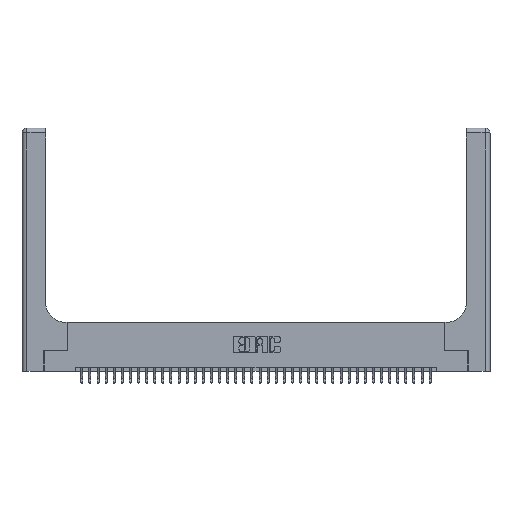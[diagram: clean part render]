
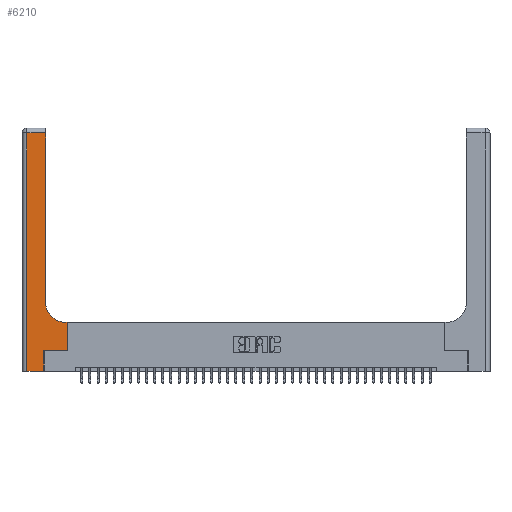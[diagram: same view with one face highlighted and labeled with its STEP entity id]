
A CAD part, top view. The second image highlights one B-rep face of the part: STEP entity #6210.
In plain terms, the highlighted planar face has unit normal (0, 0, 1).
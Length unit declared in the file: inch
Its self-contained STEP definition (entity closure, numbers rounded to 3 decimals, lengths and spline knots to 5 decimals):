
#316 = VERTEX_POINT ( 'NONE', #25435 ) ;
#557 = LINE ( 'NONE', #10463, #8726 ) ;
#2106 = CARTESIAN_POINT ( 'NONE',  ( 0.06, 3., 0.37 ) ) ;
#2370 = VECTOR ( 'NONE', #38681, 39.37008 ) ;
#2561 = VECTOR ( 'NONE', #31526, 39.37008 ) ;
#3027 = LINE ( 'NONE', #12879, #2561 ) ;
#3917 = ORIENTED_EDGE ( 'NONE', *, *, #30613, .T. ) ;
#4060 = LINE ( 'NONE', #8779, #21271 ) ;
#4466 = LINE ( 'NONE', #23834, #31785 ) ;
#4567 = DIRECTION ( 'NONE',  ( 0., 0., -1. ) ) ;
#6210 = ADVANCED_FACE ( 'NONE', ( #14023 ), #31458, .F. ) ;
#7527 = AXIS2_PLACEMENT_3D ( 'NONE', #19779, #16743, #13619 ) ;
#8027 = ORIENTED_EDGE ( 'NONE', *, *, #34618, .T. ) ;
#8530 = LINE ( 'NONE', #2106, #27703 ) ;
#8726 = VECTOR ( 'NONE', #35200, 39.37008 ) ;
#8779 = CARTESIAN_POINT ( 'NONE',  ( 0.5585, 0.25, 0.37 ) ) ;
#10171 = ORIENTED_EDGE ( 'NONE', *, *, #37333, .T. ) ;
#10463 = CARTESIAN_POINT ( 'NONE',  ( 0., 0., 0.37 ) ) ;
#10995 = DIRECTION ( 'NONE',  ( -1., 0., 0. ) ) ;
#11911 = ORIENTED_EDGE ( 'NONE', *, *, #30349, .T. ) ;
#12368 = VERTEX_POINT ( 'NONE', #21146 ) ;
#12558 = ORIENTED_EDGE ( 'NONE', *, *, #20154, .T. ) ;
#12695 = CARTESIAN_POINT ( 'NONE',  ( 0.5415, 0.6, 0.37 ) ) ;
#12879 = CARTESIAN_POINT ( 'NONE',  ( 0.269, 0., 0.37 ) ) ;
#13619 = DIRECTION ( 'NONE',  ( -1., 0., 0. ) ) ;
#14023 = FACE_OUTER_BOUND ( 'NONE', #19546, .T. ) ;
#14408 = CIRCLE ( 'NONE', #24457, 0.25 ) ;
#14654 = EDGE_CURVE ( 'NONE', #17067, #18882, #30308, .T. ) ;
#14672 = DIRECTION ( 'NONE',  ( 1., 0., 0. ) ) ;
#14797 = EDGE_CURVE ( 'NONE', #36912, #17067, #4466, .T. ) ;
#15057 = DIRECTION ( 'NONE',  ( 0., 1., 0. ) ) ;
#16743 = DIRECTION ( 'NONE',  ( 0., 0., -1. ) ) ;
#17067 = VERTEX_POINT ( 'NONE', #37466 ) ;
#17368 = VECTOR ( 'NONE', #14672, 39.37008 ) ;
#18251 = LINE ( 'NONE', #20681, #17368 ) ;
#18882 = VERTEX_POINT ( 'NONE', #34755 ) ;
#19546 = EDGE_LOOP ( 'NONE', ( #25445, #22291, #8027, #10171, #3917, #23276, #11911, #38232, #12558 ) ) ;
#19779 = CARTESIAN_POINT ( 'NONE',  ( 0., 3., 0.37 ) ) ;
#20090 = CARTESIAN_POINT ( 'NONE',  ( 0., 2.94, 0.37 ) ) ;
#20154 = EDGE_CURVE ( 'NONE', #34260, #36912, #14408, .T. ) ;
#20339 = CARTESIAN_POINT ( 'NONE',  ( 0.2915, 0.6, 0.37 ) ) ;
#20644 = EDGE_CURVE ( 'NONE', #29017, #34260, #29712, .T. ) ;
#20681 = CARTESIAN_POINT ( 'NONE',  ( 0.269, 0.25, 0.37 ) ) ;
#21146 = CARTESIAN_POINT ( 'NONE',  ( 0.06, 0., 0.37 ) ) ;
#21271 = VECTOR ( 'NONE', #15057, 39.37008 ) ;
#22291 = ORIENTED_EDGE ( 'NONE', *, *, #14654, .T. ) ;
#23117 = VECTOR ( 'NONE', #10995, 39.37008 ) ;
#23276 = ORIENTED_EDGE ( 'NONE', *, *, #38177, .T. ) ;
#23834 = CARTESIAN_POINT ( 'NONE',  ( 0.2915, 3., 0.37 ) ) ;
#24457 = AXIS2_PLACEMENT_3D ( 'NONE', #32011, #4567, #25982 ) ;
#25435 = CARTESIAN_POINT ( 'NONE',  ( 0.269, 0., 0.37 ) ) ;
#25445 = ORIENTED_EDGE ( 'NONE', *, *, #14797, .T. ) ;
#25982 = DIRECTION ( 'NONE',  ( 1., 0., 0. ) ) ;
#25990 = CARTESIAN_POINT ( 'NONE',  ( 0.5585, 0.6, 0.37 ) ) ;
#27331 = VERTEX_POINT ( 'NONE', #33329 ) ;
#27703 = VECTOR ( 'NONE', #39172, 39.37008 ) ;
#28671 = VERTEX_POINT ( 'NONE', #33487 ) ;
#29017 = VERTEX_POINT ( 'NONE', #25990 ) ;
#29712 = LINE ( 'NONE', #20339, #2370 ) ;
#29994 = DIRECTION ( 'NONE',  ( 0., 1., 0. ) ) ;
#30308 = LINE ( 'NONE', #20090, #23117 ) ;
#30349 = EDGE_CURVE ( 'NONE', #28671, #29017, #4060, .T. ) ;
#30613 = EDGE_CURVE ( 'NONE', #316, #27331, #3027, .T. ) ;
#31458 = PLANE ( 'NONE',  #7527 ) ;
#31526 = DIRECTION ( 'NONE',  ( 0., 1., 0. ) ) ;
#31785 = VECTOR ( 'NONE', #29994, 39.37008 ) ;
#32011 = CARTESIAN_POINT ( 'NONE',  ( 0.5415, 0.85, 0.37 ) ) ;
#33329 = CARTESIAN_POINT ( 'NONE',  ( 0.269, 0.25, 0.37 ) ) ;
#33487 = CARTESIAN_POINT ( 'NONE',  ( 0.5585, 0.25, 0.37 ) ) ;
#33503 = CARTESIAN_POINT ( 'NONE',  ( 0.2915, 0.85, 0.37 ) ) ;
#34260 = VERTEX_POINT ( 'NONE', #12695 ) ;
#34618 = EDGE_CURVE ( 'NONE', #18882, #12368, #8530, .T. ) ;
#34755 = CARTESIAN_POINT ( 'NONE',  ( 0.06, 2.94, 0.37 ) ) ;
#35200 = DIRECTION ( 'NONE',  ( 1., 0., 0. ) ) ;
#36912 = VERTEX_POINT ( 'NONE', #33503 ) ;
#37333 = EDGE_CURVE ( 'NONE', #12368, #316, #557, .T. ) ;
#37466 = CARTESIAN_POINT ( 'NONE',  ( 0.2915, 2.94, 0.37 ) ) ;
#38177 = EDGE_CURVE ( 'NONE', #27331, #28671, #18251, .T. ) ;
#38232 = ORIENTED_EDGE ( 'NONE', *, *, #20644, .T. ) ;
#38681 = DIRECTION ( 'NONE',  ( -1., 0., 0. ) ) ;
#39172 = DIRECTION ( 'NONE',  ( 0., -1., 0. ) ) ;
